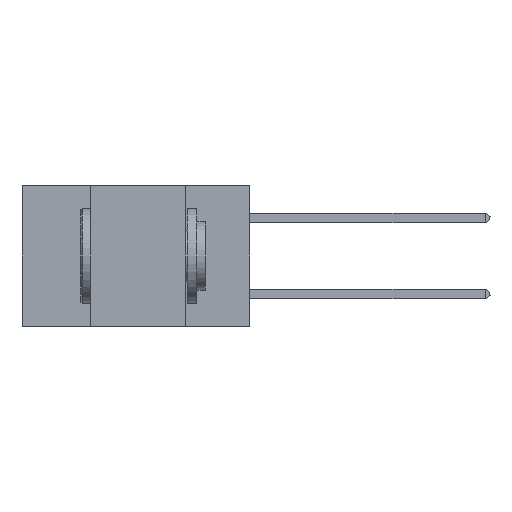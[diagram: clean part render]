
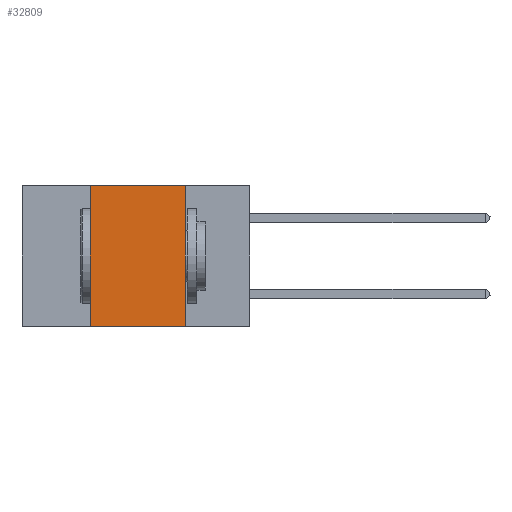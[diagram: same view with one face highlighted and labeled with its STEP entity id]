
A CAD part, left-side view. The second image highlights one B-rep face of the part: STEP entity #32809.
In plain terms, the highlighted planar face has unit normal (-1, 0, 0).
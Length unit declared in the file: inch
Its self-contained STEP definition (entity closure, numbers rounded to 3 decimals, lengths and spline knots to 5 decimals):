
#271 = LINE ( 'NONE', #23239, #1121 ) ;
#381 = CARTESIAN_POINT ( 'NONE',  ( 0., 0.6, 0. ) ) ;
#1121 = VECTOR ( 'NONE', #10227, 39.37008 ) ;
#1895 = VERTEX_POINT ( 'NONE', #7659 ) ;
#1926 = CARTESIAN_POINT ( 'NONE',  ( 0., 0.6, -0.37 ) ) ;
#2420 = AXIS2_PLACEMENT_3D ( 'NONE', #381, #18769, #3058 ) ;
#2637 = DIRECTION ( 'NONE',  ( 0., 0., -1. ) ) ;
#3058 = DIRECTION ( 'NONE',  ( 0., 0., -1. ) ) ;
#6292 = EDGE_CURVE ( 'NONE', #30517, #1895, #271, .T. ) ;
#7659 = CARTESIAN_POINT ( 'NONE',  ( 0., 0.17, 0. ) ) ;
#9500 = LINE ( 'NONE', #31389, #29468 ) ;
#10227 = DIRECTION ( 'NONE',  ( 0., -1., 0. ) ) ;
#10774 = LINE ( 'NONE', #16099, #11601 ) ;
#10840 = EDGE_LOOP ( 'NONE', ( #20217, #19244, #26001, #25648 ) ) ;
#11601 = VECTOR ( 'NONE', #31640, 39.37008 ) ;
#13220 = VERTEX_POINT ( 'NONE', #19793 ) ;
#14157 = CARTESIAN_POINT ( 'NONE',  ( 0., 0.42, -0.37 ) ) ;
#16099 = CARTESIAN_POINT ( 'NONE',  ( 0., 0.42, 0. ) ) ;
#16442 = LINE ( 'NONE', #1926, #23397 ) ;
#17074 = VERTEX_POINT ( 'NONE', #14157 ) ;
#17682 = DIRECTION ( 'NONE',  ( 0., -1., 0. ) ) ;
#18769 = DIRECTION ( 'NONE',  ( 1., 0., 0. ) ) ;
#19244 = ORIENTED_EDGE ( 'NONE', *, *, #6292, .F. ) ;
#19793 = CARTESIAN_POINT ( 'NONE',  ( 0., 0.17, -0.37 ) ) ;
#20095 = EDGE_CURVE ( 'NONE', #17074, #30517, #10774, .T. ) ;
#20217 = ORIENTED_EDGE ( 'NONE', *, *, #28763, .F. ) ;
#23239 = CARTESIAN_POINT ( 'NONE',  ( 0., 0.6, 0. ) ) ;
#23397 = VECTOR ( 'NONE', #17682, 39.37008 ) ;
#25506 = EDGE_CURVE ( 'NONE', #17074, #13220, #16442, .T. ) ;
#25539 = CARTESIAN_POINT ( 'NONE',  ( 0., 0.42, 0. ) ) ;
#25648 = ORIENTED_EDGE ( 'NONE', *, *, #25506, .T. ) ;
#26001 = ORIENTED_EDGE ( 'NONE', *, *, #20095, .F. ) ;
#26388 = FACE_OUTER_BOUND ( 'NONE', #10840, .T. ) ;
#28763 = EDGE_CURVE ( 'NONE', #1895, #13220, #9500, .T. ) ;
#29115 = PLANE ( 'NONE',  #2420 ) ;
#29468 = VECTOR ( 'NONE', #2637, 39.37008 ) ;
#30517 = VERTEX_POINT ( 'NONE', #25539 ) ;
#31389 = CARTESIAN_POINT ( 'NONE',  ( 0., 0.17, 0. ) ) ;
#31640 = DIRECTION ( 'NONE',  ( 0., 0., 1. ) ) ;
#32809 = ADVANCED_FACE ( 'NONE', ( #26388 ), #29115, .F. ) ;
